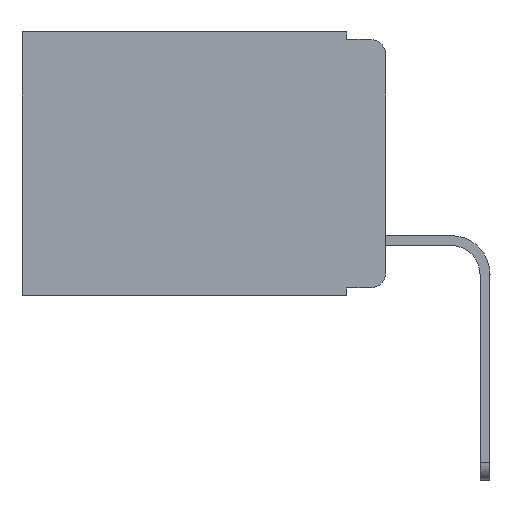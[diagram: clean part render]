
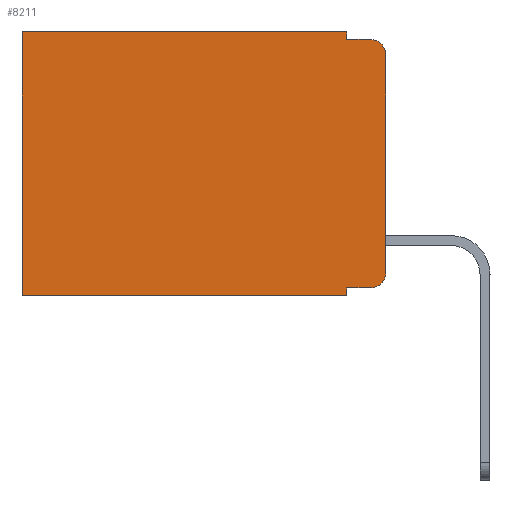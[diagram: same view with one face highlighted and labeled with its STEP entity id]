
A CAD part, left-side view. The second image highlights one B-rep face of the part: STEP entity #8211.
In plain terms, the highlighted planar face has unit normal (-1, 0, 0).
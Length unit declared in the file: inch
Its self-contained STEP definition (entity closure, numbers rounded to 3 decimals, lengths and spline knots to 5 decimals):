
#76 = ORIENTED_EDGE ( 'NONE', *, *, #20610, .F. ) ;
#644 = AXIS2_PLACEMENT_3D ( 'NONE', #6910, #9072, #8904 ) ;
#703 = CARTESIAN_POINT ( 'NONE',  ( 0.298, 0., 0. ) ) ;
#904 = EDGE_CURVE ( 'NONE', #7820, #17051, #4886, .T. ) ;
#963 = VERTEX_POINT ( 'NONE', #8502 ) ;
#1088 = ORIENTED_EDGE ( 'NONE', *, *, #22671, .T. ) ;
#1274 = CARTESIAN_POINT ( 'NONE',  ( 0.298, 0.473, 0. ) ) ;
#1680 = VECTOR ( 'NONE', #14797, 39.37008 ) ;
#2322 = DIRECTION ( 'NONE',  ( 0., 1., 0. ) ) ;
#2338 = DIRECTION ( 'NONE',  ( 0., 0., -1. ) ) ;
#2437 = VERTEX_POINT ( 'NONE', #20470 ) ;
#3459 = LINE ( 'NONE', #14676, #7068 ) ;
#3676 = CARTESIAN_POINT ( 'NONE',  ( 0.298, 0., -0.03 ) ) ;
#3899 = CIRCLE ( 'NONE', #644, 0.02 ) ;
#3923 = EDGE_LOOP ( 'NONE', ( #17674, #10275, #8915, #12555, #1088, #15442, #76, #18784, #16324, #15178 ) ) ;
#4211 = AXIS2_PLACEMENT_3D ( 'NONE', #14419, #12534, #14259 ) ;
#4865 = DIRECTION ( 'NONE',  ( 0., 0., -1. ) ) ;
#4886 = LINE ( 'NONE', #15557, #22236 ) ;
#5276 = AXIS2_PLACEMENT_3D ( 'NONE', #10795, #7065, #4865 ) ;
#5368 = CARTESIAN_POINT ( 'NONE',  ( 0.298, 0., -0.313 ) ) ;
#5780 = CARTESIAN_POINT ( 'NONE',  ( 0.298, 0.02, -0.333 ) ) ;
#6012 = CARTESIAN_POINT ( 'NONE',  ( 0.298, 0.051, -0.343 ) ) ;
#6910 = CARTESIAN_POINT ( 'NONE',  ( 0.298, 0.02, -0.313 ) ) ;
#7065 = DIRECTION ( 'NONE',  ( -1., 0., 0. ) ) ;
#7068 = VECTOR ( 'NONE', #16768, 39.37008 ) ;
#7820 = VERTEX_POINT ( 'NONE', #1274 ) ;
#7999 = VERTEX_POINT ( 'NONE', #6012 ) ;
#8211 = ADVANCED_FACE ( 'NONE', ( #12504 ), #20050, .F. ) ;
#8502 = CARTESIAN_POINT ( 'NONE',  ( 0.298, 0.051, 0. ) ) ;
#8904 = DIRECTION ( 'NONE',  ( 0., 0., -1. ) ) ;
#8915 = ORIENTED_EDGE ( 'NONE', *, *, #21125, .F. ) ;
#9072 = DIRECTION ( 'NONE',  ( -1., 0., 0. ) ) ;
#9181 = LINE ( 'NONE', #703, #13627 ) ;
#9481 = EDGE_CURVE ( 'NONE', #963, #21901, #3459, .T. ) ;
#10028 = LINE ( 'NONE', #23319, #12988 ) ;
#10275 = ORIENTED_EDGE ( 'NONE', *, *, #24068, .T. ) ;
#10795 = CARTESIAN_POINT ( 'NONE',  ( 0.298, 0.02, -0.03 ) ) ;
#10847 = DIRECTION ( 'NONE',  ( 0., -1., 0. ) ) ;
#10967 = LINE ( 'NONE', #10994, #1680 ) ;
#10994 = CARTESIAN_POINT ( 'NONE',  ( 0.298, 0.051, -0.01 ) ) ;
#11351 = EDGE_CURVE ( 'NONE', #14280, #22603, #24608, .T. ) ;
#12039 = CIRCLE ( 'NONE', #5276, 0.02 ) ;
#12504 = FACE_OUTER_BOUND ( 'NONE', #3923, .T. ) ;
#12534 = DIRECTION ( 'NONE',  ( 1., 0., 0. ) ) ;
#12555 = ORIENTED_EDGE ( 'NONE', *, *, #9481, .F. ) ;
#12967 = EDGE_CURVE ( 'NONE', #20706, #15805, #9181, .T. ) ;
#12988 = VECTOR ( 'NONE', #2322, 39.37008 ) ;
#13627 = VECTOR ( 'NONE', #14038, 39.37008 ) ;
#14038 = DIRECTION ( 'NONE',  ( 0., 0., -1. ) ) ;
#14243 = LINE ( 'NONE', #22648, #15759 ) ;
#14259 = DIRECTION ( 'NONE',  ( 0., 0., -1. ) ) ;
#14280 = VERTEX_POINT ( 'NONE', #24513 ) ;
#14419 = CARTESIAN_POINT ( 'NONE',  ( 0.298, 0., 0. ) ) ;
#14676 = CARTESIAN_POINT ( 'NONE',  ( 0.298, 0.051, 0. ) ) ;
#14797 = DIRECTION ( 'NONE',  ( 0., -1., 0. ) ) ;
#15178 = ORIENTED_EDGE ( 'NONE', *, *, #16944, .T. ) ;
#15442 = ORIENTED_EDGE ( 'NONE', *, *, #904, .T. ) ;
#15557 = CARTESIAN_POINT ( 'NONE',  ( 0.298, 0.473, 0. ) ) ;
#15567 = VECTOR ( 'NONE', #10847, 39.37008 ) ;
#15759 = VECTOR ( 'NONE', #22811, 39.37008 ) ;
#15805 = VERTEX_POINT ( 'NONE', #5368 ) ;
#16324 = ORIENTED_EDGE ( 'NONE', *, *, #11351, .T. ) ;
#16379 = LINE ( 'NONE', #21661, #23325 ) ;
#16768 = DIRECTION ( 'NONE',  ( 0., 0., -1. ) ) ;
#16944 = EDGE_CURVE ( 'NONE', #22603, #15805, #3899, .T. ) ;
#17051 = VERTEX_POINT ( 'NONE', #24536 ) ;
#17491 = DIRECTION ( 'NONE',  ( 0., 0., -1. ) ) ;
#17674 = ORIENTED_EDGE ( 'NONE', *, *, #12967, .F. ) ;
#18510 = CARTESIAN_POINT ( 'NONE',  ( 0.298, 0.051, -0.333 ) ) ;
#18784 = ORIENTED_EDGE ( 'NONE', *, *, #19938, .F. ) ;
#19938 = EDGE_CURVE ( 'NONE', #14280, #7999, #16379, .T. ) ;
#20050 = PLANE ( 'NONE',  #4211 ) ;
#20470 = CARTESIAN_POINT ( 'NONE',  ( 0.298, 0.02, -0.01 ) ) ;
#20610 = EDGE_CURVE ( 'NONE', #7999, #17051, #14243, .T. ) ;
#20706 = VERTEX_POINT ( 'NONE', #3676 ) ;
#21018 = CARTESIAN_POINT ( 'NONE',  ( 0.298, 0.051, -0.01 ) ) ;
#21125 = EDGE_CURVE ( 'NONE', #21901, #2437, #10967, .T. ) ;
#21661 = CARTESIAN_POINT ( 'NONE',  ( 0.298, 0.051, 0. ) ) ;
#21901 = VERTEX_POINT ( 'NONE', #21018 ) ;
#22236 = VECTOR ( 'NONE', #17491, 39.37008 ) ;
#22603 = VERTEX_POINT ( 'NONE', #5780 ) ;
#22648 = CARTESIAN_POINT ( 'NONE',  ( 0.298, 0., -0.343 ) ) ;
#22671 = EDGE_CURVE ( 'NONE', #963, #7820, #10028, .T. ) ;
#22811 = DIRECTION ( 'NONE',  ( 0., 1., 0. ) ) ;
#23319 = CARTESIAN_POINT ( 'NONE',  ( 0.298, 0., 0. ) ) ;
#23325 = VECTOR ( 'NONE', #2338, 39.37008 ) ;
#24068 = EDGE_CURVE ( 'NONE', #20706, #2437, #12039, .T. ) ;
#24513 = CARTESIAN_POINT ( 'NONE',  ( 0.298, 0.051, -0.333 ) ) ;
#24536 = CARTESIAN_POINT ( 'NONE',  ( 0.298, 0.473, -0.343 ) ) ;
#24608 = LINE ( 'NONE', #18510, #15567 ) ;
